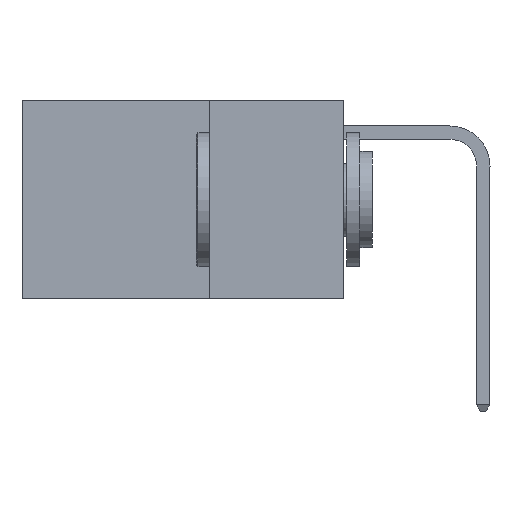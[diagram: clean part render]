
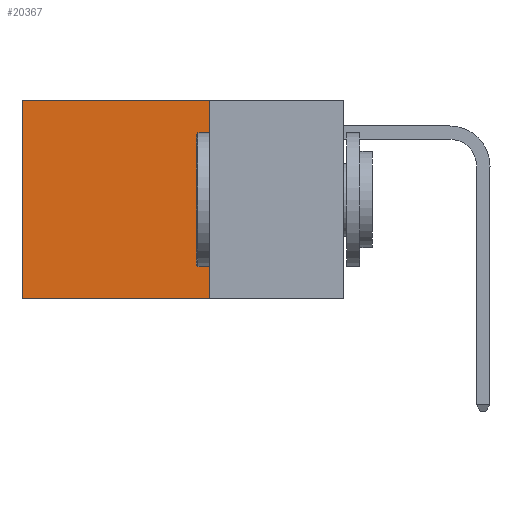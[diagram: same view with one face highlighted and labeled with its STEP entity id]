
A CAD part, left-side view. The second image highlights one B-rep face of the part: STEP entity #20367.
In plain terms, the highlighted planar face has unit normal (-1, 0, 0).
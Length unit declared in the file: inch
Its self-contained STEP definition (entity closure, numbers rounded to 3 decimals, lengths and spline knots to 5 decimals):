
#185 = CARTESIAN_POINT ( 'NONE',  ( 0.2625, 0.25, -0.37 ) ) ;
#327 = EDGE_CURVE ( 'NONE', #16817, #1971, #17838, .T. ) ;
#1025 = CARTESIAN_POINT ( 'NONE',  ( 0.2625, 0.25, -0.37 ) ) ;
#1454 = FACE_OUTER_BOUND ( 'NONE', #4959, .T. ) ;
#1971 = VERTEX_POINT ( 'NONE', #20665 ) ;
#3165 = EDGE_CURVE ( 'NONE', #16817, #23300, #18164, .T. ) ;
#3821 = CARTESIAN_POINT ( 'NONE',  ( 0.2625, 0.25, 0. ) ) ;
#4567 = CARTESIAN_POINT ( 'NONE',  ( 0.2625, 0.25, 0. ) ) ;
#4898 = DIRECTION ( 'NONE',  ( 0., 0., -1. ) ) ;
#4959 = EDGE_LOOP ( 'NONE', ( #16428, #18463, #11563, #12942 ) ) ;
#8336 = AXIS2_PLACEMENT_3D ( 'NONE', #3821, #20438, #9395 ) ;
#9395 = DIRECTION ( 'NONE',  ( 0., 0., -1. ) ) ;
#10842 = VECTOR ( 'NONE', #13925, 39.37008 ) ;
#11563 = ORIENTED_EDGE ( 'NONE', *, *, #3165, .F. ) ;
#11928 = CARTESIAN_POINT ( 'NONE',  ( 0.2625, 0.25, 0. ) ) ;
#12721 = VECTOR ( 'NONE', #17909, 39.37008 ) ;
#12942 = ORIENTED_EDGE ( 'NONE', *, *, #327, .T. ) ;
#12966 = VECTOR ( 'NONE', #21900, 39.37008 ) ;
#13925 = DIRECTION ( 'NONE',  ( 0., 1., 0. ) ) ;
#14625 = LINE ( 'NONE', #17778, #18958 ) ;
#16114 = VERTEX_POINT ( 'NONE', #19397 ) ;
#16428 = ORIENTED_EDGE ( 'NONE', *, *, #21957, .T. ) ;
#16723 = PLANE ( 'NONE',  #8336 ) ;
#16817 = VERTEX_POINT ( 'NONE', #11928 ) ;
#17778 = CARTESIAN_POINT ( 'NONE',  ( 0.2625, 0.6, 0. ) ) ;
#17838 = LINE ( 'NONE', #4567, #12966 ) ;
#17909 = DIRECTION ( 'NONE',  ( 0., 0., -1. ) ) ;
#18031 = CARTESIAN_POINT ( 'NONE',  ( 0.2625, 0.25, 0. ) ) ;
#18164 = LINE ( 'NONE', #18031, #12721 ) ;
#18186 = EDGE_CURVE ( 'NONE', #23300, #16114, #23777, .T. ) ;
#18463 = ORIENTED_EDGE ( 'NONE', *, *, #18186, .F. ) ;
#18958 = VECTOR ( 'NONE', #4898, 39.37008 ) ;
#19397 = CARTESIAN_POINT ( 'NONE',  ( 0.2625, 0.6, -0.37 ) ) ;
#20367 = ADVANCED_FACE ( 'NONE', ( #1454 ), #16723, .F. ) ;
#20438 = DIRECTION ( 'NONE',  ( 1., 0., 0. ) ) ;
#20665 = CARTESIAN_POINT ( 'NONE',  ( 0.2625, 0.6, 0. ) ) ;
#21900 = DIRECTION ( 'NONE',  ( 0., 1., 0. ) ) ;
#21957 = EDGE_CURVE ( 'NONE', #1971, #16114, #14625, .T. ) ;
#23300 = VERTEX_POINT ( 'NONE', #185 ) ;
#23777 = LINE ( 'NONE', #1025, #10842 ) ;
